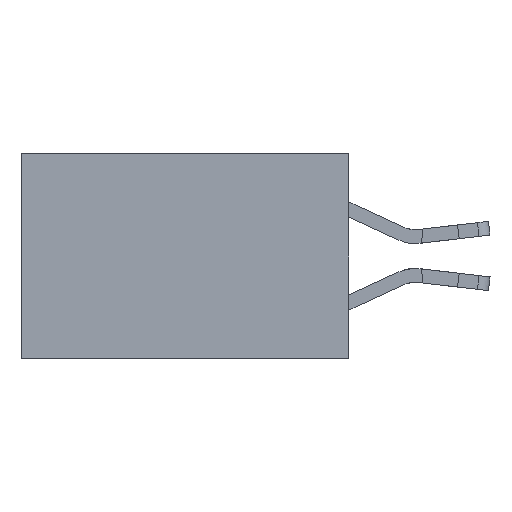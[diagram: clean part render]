
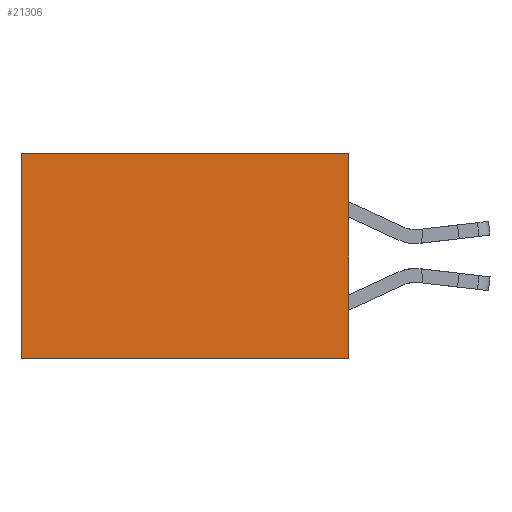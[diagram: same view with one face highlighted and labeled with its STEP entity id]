
A CAD part, left-side view. The second image highlights one B-rep face of the part: STEP entity #21306.
In plain terms, the highlighted planar face has unit normal (-1, 0, 0).
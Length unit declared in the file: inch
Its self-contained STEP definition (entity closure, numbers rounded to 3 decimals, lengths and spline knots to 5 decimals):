
#1766 = LINE ( 'NONE', #22275, #6957 ) ;
#1979 = CARTESIAN_POINT ( 'NONE',  ( 0.277, 0., 0. ) ) ;
#2358 = DIRECTION ( 'NONE',  ( 1., 0., 0. ) ) ;
#2628 = VECTOR ( 'NONE', #5444, 39.37008 ) ;
#2978 = FACE_OUTER_BOUND ( 'NONE', #8902, .T. ) ;
#4146 = VECTOR ( 'NONE', #19649, 39.37008 ) ;
#4627 = DIRECTION ( 'NONE',  ( 0., 0., -1. ) ) ;
#5444 = DIRECTION ( 'NONE',  ( 0., 0., -1. ) ) ;
#6267 = VERTEX_POINT ( 'NONE', #16172 ) ;
#6957 = VECTOR ( 'NONE', #4627, 39.37008 ) ;
#8034 = CARTESIAN_POINT ( 'NONE',  ( 0.277, 0., -0.37 ) ) ;
#8902 = EDGE_LOOP ( 'NONE', ( #26200, #24606, #19086, #25681 ) ) ;
#9830 = CARTESIAN_POINT ( 'NONE',  ( 0.277, 0., 0. ) ) ;
#10305 = VECTOR ( 'NONE', #23436, 39.37008 ) ;
#15598 = PLANE ( 'NONE',  #20305 ) ;
#16172 = CARTESIAN_POINT ( 'NONE',  ( 0.277, 0., -0.37 ) ) ;
#17818 = DIRECTION ( 'NONE',  ( 0., 0., -1. ) ) ;
#18130 = VERTEX_POINT ( 'NONE', #9830 ) ;
#18626 = EDGE_CURVE ( 'NONE', #18130, #6267, #1766, .T. ) ;
#19086 = ORIENTED_EDGE ( 'NONE', *, *, #18626, .F. ) ;
#19174 = EDGE_CURVE ( 'NONE', #18130, #27241, #21754, .T. ) ;
#19538 = VERTEX_POINT ( 'NONE', #27371 ) ;
#19649 = DIRECTION ( 'NONE',  ( 0., 1., 0. ) ) ;
#20265 = EDGE_CURVE ( 'NONE', #6267, #19538, #27157, .T. ) ;
#20305 = AXIS2_PLACEMENT_3D ( 'NONE', #26528, #2358, #17818 ) ;
#20648 = CARTESIAN_POINT ( 'NONE',  ( 0.277, 0.59, 0. ) ) ;
#21306 = ADVANCED_FACE ( 'NONE', ( #2978 ), #15598, .F. ) ;
#21754 = LINE ( 'NONE', #1979, #4146 ) ;
#22275 = CARTESIAN_POINT ( 'NONE',  ( 0.277, 0., -0.37 ) ) ;
#22612 = EDGE_CURVE ( 'NONE', #27241, #19538, #27438, .T. ) ;
#23436 = DIRECTION ( 'NONE',  ( 0., 1., 0. ) ) ;
#24606 = ORIENTED_EDGE ( 'NONE', *, *, #20265, .F. ) ;
#25681 = ORIENTED_EDGE ( 'NONE', *, *, #19174, .T. ) ;
#26200 = ORIENTED_EDGE ( 'NONE', *, *, #22612, .T. ) ;
#26528 = CARTESIAN_POINT ( 'NONE',  ( 0.277, 0., -0.37 ) ) ;
#27157 = LINE ( 'NONE', #8034, #10305 ) ;
#27241 = VERTEX_POINT ( 'NONE', #20648 ) ;
#27369 = CARTESIAN_POINT ( 'NONE',  ( 0.277, 0.59, -0.37 ) ) ;
#27371 = CARTESIAN_POINT ( 'NONE',  ( 0.277, 0.59, -0.37 ) ) ;
#27438 = LINE ( 'NONE', #27369, #2628 ) ;
